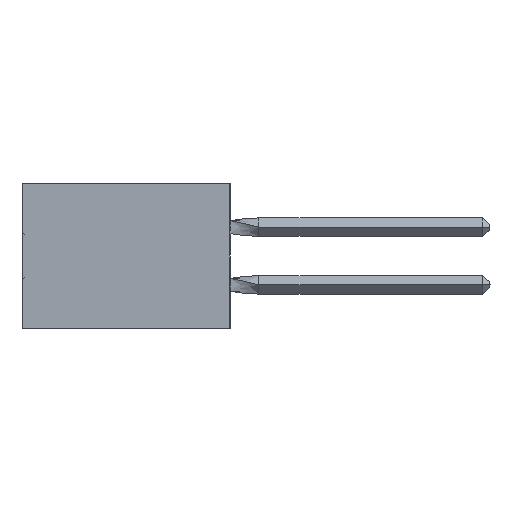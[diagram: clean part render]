
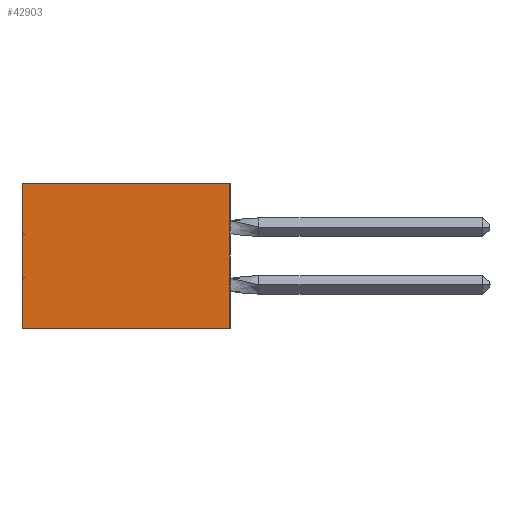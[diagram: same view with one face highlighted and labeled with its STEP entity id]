
A CAD part, left-side view. The second image highlights one B-rep face of the part: STEP entity #42903.
In plain terms, the highlighted planar face has unit normal (-1, 0, 0).
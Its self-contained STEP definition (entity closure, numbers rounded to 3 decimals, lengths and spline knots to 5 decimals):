
#7347 = DIRECTION ( 'NONE',  ( 0., 0., -1. ) ) ;
#7545 = CARTESIAN_POINT ( 'NONE',  ( 0.305, 0., -0.5 ) ) ;
#8135 = DIRECTION ( 'NONE',  ( 1., 0., 0. ) ) ;
#8907 = VECTOR ( 'NONE', #31372, 39.37008 ) ;
#10410 = VERTEX_POINT ( 'NONE', #52878 ) ;
#11003 = ORIENTED_EDGE ( 'NONE', *, *, #19549, .F. ) ;
#12596 = CARTESIAN_POINT ( 'NONE',  ( 0.305, 0., 0. ) ) ;
#12931 = DIRECTION ( 'NONE',  ( 0., 0., -1. ) ) ;
#13204 = LINE ( 'NONE', #35600, #48960 ) ;
#13411 = CARTESIAN_POINT ( 'NONE',  ( 0.305, 0., -0.5 ) ) ;
#15107 = VERTEX_POINT ( 'NONE', #39400 ) ;
#16323 = EDGE_CURVE ( 'NONE', #16837, #15107, #13204, .T. ) ;
#16837 = VERTEX_POINT ( 'NONE', #13411 ) ;
#19549 = EDGE_CURVE ( 'NONE', #50600, #16837, #41997, .T. ) ;
#21239 = LINE ( 'NONE', #21971, #8907 ) ;
#21971 = CARTESIAN_POINT ( 'NONE',  ( 0.305, 0., 0. ) ) ;
#23120 = VECTOR ( 'NONE', #51664, 39.37008 ) ;
#31107 = PLANE ( 'NONE',  #43490 ) ;
#31372 = DIRECTION ( 'NONE',  ( 0., 1., 0. ) ) ;
#33708 = CARTESIAN_POINT ( 'NONE',  ( 0.305, 0., -0.5 ) ) ;
#34585 = ORIENTED_EDGE ( 'NONE', *, *, #45647, .T. ) ;
#35445 = VECTOR ( 'NONE', #12931, 39.37008 ) ;
#35600 = CARTESIAN_POINT ( 'NONE',  ( 0.305, 0., -0.5 ) ) ;
#39400 = CARTESIAN_POINT ( 'NONE',  ( 0.305, 0.72, -0.5 ) ) ;
#41492 = EDGE_CURVE ( 'NONE', #10410, #15107, #48044, .T. ) ;
#41997 = LINE ( 'NONE', #33708, #35445 ) ;
#42903 = ADVANCED_FACE ( 'NONE', ( #43570 ), #31107, .F. ) ;
#43490 = AXIS2_PLACEMENT_3D ( 'NONE', #7545, #8135, #7347 ) ;
#43570 = FACE_OUTER_BOUND ( 'NONE', #50742, .T. ) ;
#45647 = EDGE_CURVE ( 'NONE', #50600, #10410, #21239, .T. ) ;
#46824 = CARTESIAN_POINT ( 'NONE',  ( 0.305, 0.72, -0.5 ) ) ;
#48044 = LINE ( 'NONE', #46824, #23120 ) ;
#48615 = ORIENTED_EDGE ( 'NONE', *, *, #16323, .F. ) ;
#48960 = VECTOR ( 'NONE', #53721, 39.37008 ) ;
#49926 = ORIENTED_EDGE ( 'NONE', *, *, #41492, .T. ) ;
#50600 = VERTEX_POINT ( 'NONE', #12596 ) ;
#50742 = EDGE_LOOP ( 'NONE', ( #49926, #48615, #11003, #34585 ) ) ;
#51664 = DIRECTION ( 'NONE',  ( 0., 0., -1. ) ) ;
#52878 = CARTESIAN_POINT ( 'NONE',  ( 0.305, 0.72, 0. ) ) ;
#53721 = DIRECTION ( 'NONE',  ( 0., 1., 0. ) ) ;
